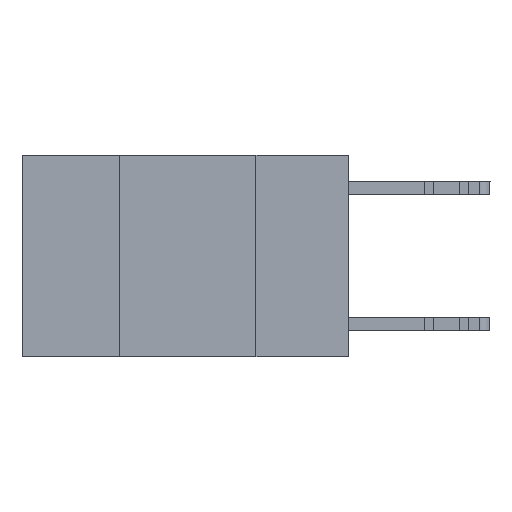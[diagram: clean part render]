
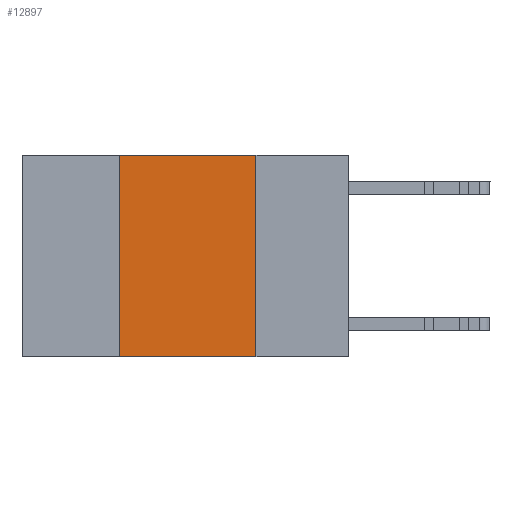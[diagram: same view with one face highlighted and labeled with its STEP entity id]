
A CAD part, left-side view. The second image highlights one B-rep face of the part: STEP entity #12897.
In plain terms, the highlighted planar face has unit normal (-1, 0, 0).
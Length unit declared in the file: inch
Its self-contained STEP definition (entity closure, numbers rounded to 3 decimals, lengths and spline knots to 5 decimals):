
#340 = LINE ( 'NONE', #19151, #9033 ) ;
#395 = EDGE_LOOP ( 'NONE', ( #19416, #14431, #28307, #21902 ) ) ;
#1666 = VECTOR ( 'NONE', #18954, 39.37008 ) ;
#3531 = CARTESIAN_POINT ( 'NONE',  ( 0., 0.42, 0. ) ) ;
#4482 = CARTESIAN_POINT ( 'NONE',  ( 0., 0.17, 0. ) ) ;
#5489 = CARTESIAN_POINT ( 'NONE',  ( 0., 0.6, 0. ) ) ;
#7617 = DIRECTION ( 'NONE',  ( 1., 0., 0. ) ) ;
#9033 = VECTOR ( 'NONE', #9630, 39.37008 ) ;
#9630 = DIRECTION ( 'NONE',  ( 0., -1., 0. ) ) ;
#9907 = FACE_OUTER_BOUND ( 'NONE', #395, .T. ) ;
#12160 = PLANE ( 'NONE',  #20451 ) ;
#12496 = EDGE_CURVE ( 'NONE', #13029, #26573, #16644, .T. ) ;
#12897 = ADVANCED_FACE ( 'NONE', ( #9907 ), #12160, .F. ) ;
#13029 = VERTEX_POINT ( 'NONE', #21006 ) ;
#13618 = VERTEX_POINT ( 'NONE', #17731 ) ;
#13678 = VECTOR ( 'NONE', #27758, 39.37008 ) ;
#14431 = ORIENTED_EDGE ( 'NONE', *, *, #19015, .F. ) ;
#14767 = LINE ( 'NONE', #3531, #15338 ) ;
#14894 = VERTEX_POINT ( 'NONE', #4482 ) ;
#14920 = DIRECTION ( 'NONE',  ( 0., 0., 1. ) ) ;
#14970 = CARTESIAN_POINT ( 'NONE',  ( 0., 0.17, -0.37 ) ) ;
#15338 = VECTOR ( 'NONE', #14920, 39.37008 ) ;
#16569 = DIRECTION ( 'NONE',  ( 0., 0., -1. ) ) ;
#16644 = LINE ( 'NONE', #16789, #13678 ) ;
#16789 = CARTESIAN_POINT ( 'NONE',  ( 0., 0.6, -0.37 ) ) ;
#17390 = EDGE_CURVE ( 'NONE', #14894, #26573, #18363, .T. ) ;
#17731 = CARTESIAN_POINT ( 'NONE',  ( 0., 0.42, 0. ) ) ;
#18363 = LINE ( 'NONE', #27653, #1666 ) ;
#18954 = DIRECTION ( 'NONE',  ( 0., 0., -1. ) ) ;
#19015 = EDGE_CURVE ( 'NONE', #13618, #14894, #340, .T. ) ;
#19057 = EDGE_CURVE ( 'NONE', #13029, #13618, #14767, .T. ) ;
#19151 = CARTESIAN_POINT ( 'NONE',  ( 0., 0.6, 0. ) ) ;
#19416 = ORIENTED_EDGE ( 'NONE', *, *, #17390, .F. ) ;
#20451 = AXIS2_PLACEMENT_3D ( 'NONE', #5489, #7617, #16569 ) ;
#21006 = CARTESIAN_POINT ( 'NONE',  ( 0., 0.42, -0.37 ) ) ;
#21902 = ORIENTED_EDGE ( 'NONE', *, *, #12496, .T. ) ;
#26573 = VERTEX_POINT ( 'NONE', #14970 ) ;
#27653 = CARTESIAN_POINT ( 'NONE',  ( 0., 0.17, 0. ) ) ;
#27758 = DIRECTION ( 'NONE',  ( 0., -1., 0. ) ) ;
#28307 = ORIENTED_EDGE ( 'NONE', *, *, #19057, .F. ) ;
